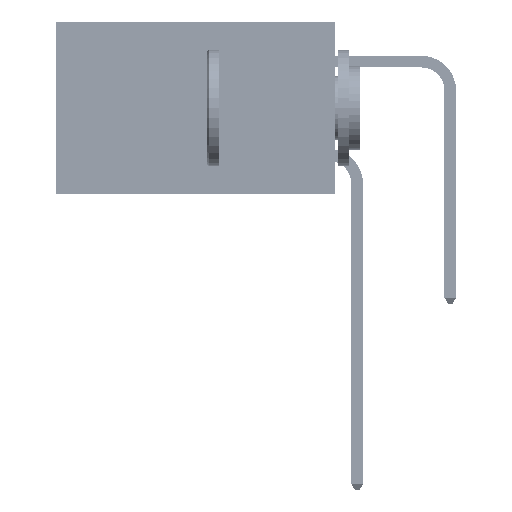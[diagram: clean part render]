
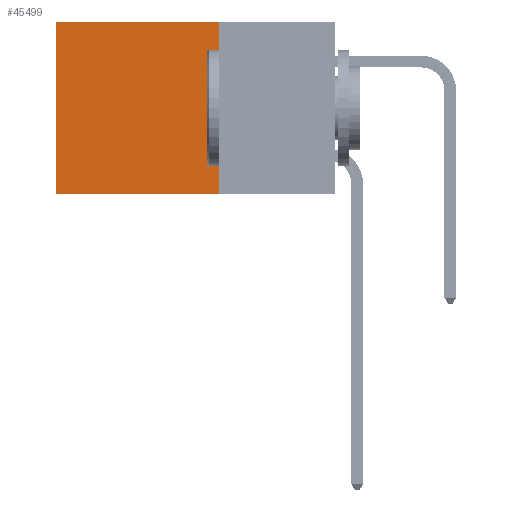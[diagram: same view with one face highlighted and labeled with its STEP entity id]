
A CAD part, left-side view. The second image highlights one B-rep face of the part: STEP entity #45499.
In plain terms, the highlighted planar face has unit normal (-1, 0, 0).
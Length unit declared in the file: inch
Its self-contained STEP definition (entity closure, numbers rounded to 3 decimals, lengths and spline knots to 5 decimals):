
#1223 = CARTESIAN_POINT ( 'NONE',  ( 0.2875, 0.25, -0.37 ) ) ;
#1303 = CARTESIAN_POINT ( 'NONE',  ( 0.2875, 0.25, -0.37 ) ) ;
#4465 = DIRECTION ( 'NONE',  ( 1., 0., 0. ) ) ;
#6605 = DIRECTION ( 'NONE',  ( 0., 1., 0. ) ) ;
#6646 = LINE ( 'NONE', #46068, #48407 ) ;
#7312 = ORIENTED_EDGE ( 'NONE', *, *, #49253, .T. ) ;
#7952 = VERTEX_POINT ( 'NONE', #1303 ) ;
#8187 = CARTESIAN_POINT ( 'NONE',  ( 0.2875, 0.6, 0. ) ) ;
#12149 = ORIENTED_EDGE ( 'NONE', *, *, #14352, .T. ) ;
#12199 = ORIENTED_EDGE ( 'NONE', *, *, #37975, .F. ) ;
#13331 = VERTEX_POINT ( 'NONE', #15457 ) ;
#14352 = EDGE_CURVE ( 'NONE', #20790, #20202, #6646, .T. ) ;
#15089 = VECTOR ( 'NONE', #21389, 39.37008 ) ;
#15457 = CARTESIAN_POINT ( 'NONE',  ( 0.2875, 0.6, -0.37 ) ) ;
#15953 = PLANE ( 'NONE',  #27314 ) ;
#16114 = EDGE_LOOP ( 'NONE', ( #7312, #22914, #12199, #12149 ) ) ;
#20202 = VERTEX_POINT ( 'NONE', #8187 ) ;
#20790 = VERTEX_POINT ( 'NONE', #30876 ) ;
#21019 = EDGE_CURVE ( 'NONE', #7952, #13331, #49781, .T. ) ;
#21204 = FACE_OUTER_BOUND ( 'NONE', #16114, .T. ) ;
#21389 = DIRECTION ( 'NONE',  ( 0., 0., -1. ) ) ;
#22914 = ORIENTED_EDGE ( 'NONE', *, *, #21019, .F. ) ;
#23599 = DIRECTION ( 'NONE',  ( 0., 0., -1. ) ) ;
#27314 = AXIS2_PLACEMENT_3D ( 'NONE', #39784, #4465, #43406 ) ;
#30876 = CARTESIAN_POINT ( 'NONE',  ( 0.2875, 0.25, 0. ) ) ;
#32700 = DIRECTION ( 'NONE',  ( 0., 1., 0. ) ) ;
#37975 = EDGE_CURVE ( 'NONE', #20790, #7952, #47675, .T. ) ;
#39784 = CARTESIAN_POINT ( 'NONE',  ( 0.2875, 0.25, 0. ) ) ;
#40764 = CARTESIAN_POINT ( 'NONE',  ( 0.2875, 0.25, 0. ) ) ;
#42345 = VECTOR ( 'NONE', #32700, 39.37008 ) ;
#42663 = VECTOR ( 'NONE', #23599, 39.37008 ) ;
#43406 = DIRECTION ( 'NONE',  ( 0., 0., -1. ) ) ;
#45499 = ADVANCED_FACE ( 'NONE', ( #21204 ), #15953, .F. ) ;
#45743 = LINE ( 'NONE', #50348, #42663 ) ;
#46068 = CARTESIAN_POINT ( 'NONE',  ( 0.2875, 0.25, 0. ) ) ;
#47675 = LINE ( 'NONE', #40764, #15089 ) ;
#48407 = VECTOR ( 'NONE', #6605, 39.37008 ) ;
#49253 = EDGE_CURVE ( 'NONE', #20202, #13331, #45743, .T. ) ;
#49781 = LINE ( 'NONE', #1223, #42345 ) ;
#50348 = CARTESIAN_POINT ( 'NONE',  ( 0.2875, 0.6, 0. ) ) ;
